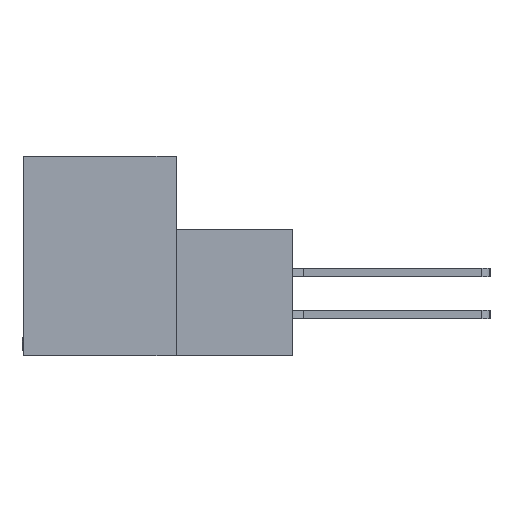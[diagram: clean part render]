
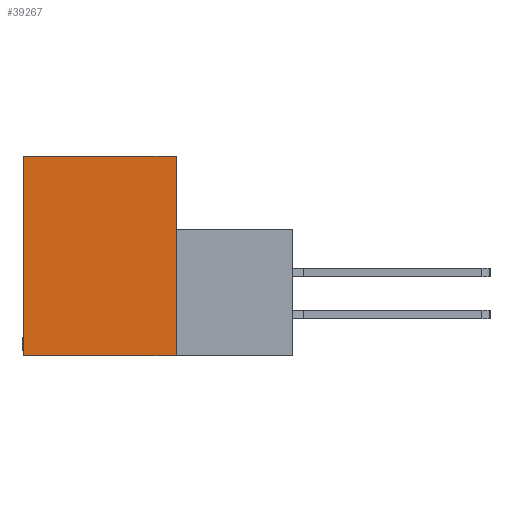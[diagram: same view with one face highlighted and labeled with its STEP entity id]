
A CAD part, left-side view. The second image highlights one B-rep face of the part: STEP entity #39267.
In plain terms, the highlighted planar face has unit normal (-1, 0, 0).
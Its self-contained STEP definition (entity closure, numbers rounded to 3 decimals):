
#35 = EDGE_LOOP ( 'NONE', ( #24415, #17802, #28259, #20020 ) ) ;
#3888 = LINE ( 'NONE', #49652, #23706 ) ;
#5631 = VERTEX_POINT ( 'NONE', #21130 ) ;
#7636 = VECTOR ( 'NONE', #50405, 1000. ) ;
#8736 = CARTESIAN_POINT ( 'NONE',  ( 0., 11.506, 0. ) ) ;
#8792 = CARTESIAN_POINT ( 'NONE',  ( 0., 0., 0. ) ) ;
#11937 = CARTESIAN_POINT ( 'NONE',  ( 0., 0., -15.088 ) ) ;
#12561 = DIRECTION ( 'NONE',  ( 0., -1., 0. ) ) ;
#13626 = EDGE_CURVE ( 'NONE', #23390, #5631, #48958, .T. ) ;
#15646 = EDGE_CURVE ( 'NONE', #33749, #26461, #36957, .T. ) ;
#17440 = CARTESIAN_POINT ( 'NONE',  ( 0., -8.814, -15.088 ) ) ;
#17802 = ORIENTED_EDGE ( 'NONE', *, *, #27294, .F. ) ;
#20020 = ORIENTED_EDGE ( 'NONE', *, *, #20107, .F. ) ;
#20107 = EDGE_CURVE ( 'NONE', #5631, #33749, #3888, .T. ) ;
#20543 = VECTOR ( 'NONE', #25359, 1000. ) ;
#21130 = CARTESIAN_POINT ( 'NONE',  ( 0., 11.506, -15.088 ) ) ;
#22204 = AXIS2_PLACEMENT_3D ( 'NONE', #8792, #48351, #36409 ) ;
#22315 = CARTESIAN_POINT ( 'NONE',  ( 0., 11.506, 0. ) ) ;
#23390 = VERTEX_POINT ( 'NONE', #11937 ) ;
#23706 = VECTOR ( 'NONE', #41368, 1000. ) ;
#24415 = ORIENTED_EDGE ( 'NONE', *, *, #13626, .F. ) ;
#25359 = DIRECTION ( 'NONE',  ( 0., 1., 0. ) ) ;
#25866 = VECTOR ( 'NONE', #12561, 1000. ) ;
#26461 = VERTEX_POINT ( 'NONE', #36323 ) ;
#27294 = EDGE_CURVE ( 'NONE', #26461, #23390, #47195, .T. ) ;
#28259 = ORIENTED_EDGE ( 'NONE', *, *, #15646, .F. ) ;
#33749 = VERTEX_POINT ( 'NONE', #22315 ) ;
#36323 = CARTESIAN_POINT ( 'NONE',  ( 0., 0., 0. ) ) ;
#36409 = DIRECTION ( 'NONE',  ( 0., 0., -1. ) ) ;
#36957 = LINE ( 'NONE', #8736, #25866 ) ;
#38491 = CARTESIAN_POINT ( 'NONE',  ( 0., 0., 0. ) ) ;
#39267 = ADVANCED_FACE ( 'NONE', ( #42688 ), #44040, .F. ) ;
#41368 = DIRECTION ( 'NONE',  ( 0., 0., 1. ) ) ;
#42688 = FACE_OUTER_BOUND ( 'NONE', #35, .T. ) ;
#44040 = PLANE ( 'NONE',  #22204 ) ;
#47195 = LINE ( 'NONE', #38491, #7636 ) ;
#48351 = DIRECTION ( 'NONE',  ( 1., 0., 0. ) ) ;
#48958 = LINE ( 'NONE', #17440, #20543 ) ;
#49652 = CARTESIAN_POINT ( 'NONE',  ( 0., 11.506, -15.088 ) ) ;
#50405 = DIRECTION ( 'NONE',  ( 0., 0., -1. ) ) ;
